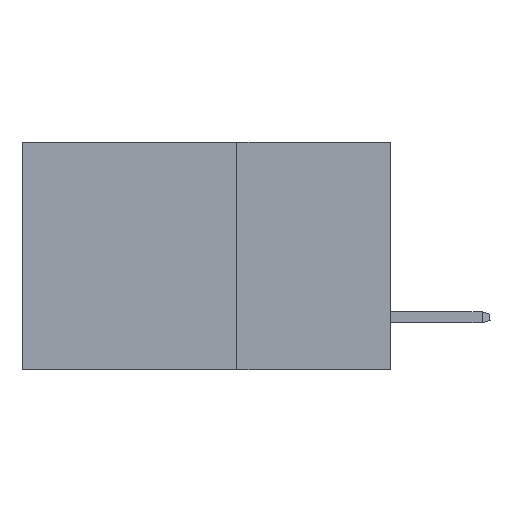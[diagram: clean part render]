
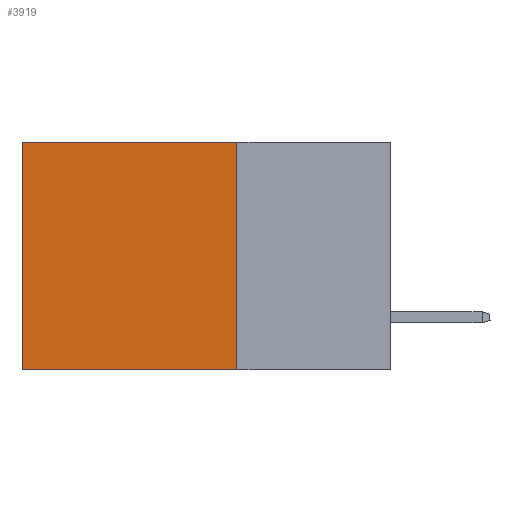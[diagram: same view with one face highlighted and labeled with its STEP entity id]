
A CAD part, left-side view. The second image highlights one B-rep face of the part: STEP entity #3919.
In plain terms, the highlighted planar face has unit normal (-1, 0, 0).
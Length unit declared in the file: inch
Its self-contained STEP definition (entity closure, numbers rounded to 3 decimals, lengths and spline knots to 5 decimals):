
#360 = VECTOR ( 'NONE', #10795, 39.37008 ) ;
#490 = VERTEX_POINT ( 'NONE', #14392 ) ;
#1005 = DIRECTION ( 'NONE',  ( 0., 1., 0. ) ) ;
#1108 = ORIENTED_EDGE ( 'NONE', *, *, #11554, .T. ) ;
#1301 = CARTESIAN_POINT ( 'NONE',  ( 0.2875, 0.6, 0. ) ) ;
#2172 = CARTESIAN_POINT ( 'NONE',  ( 0.2875, 0.25, -0.37 ) ) ;
#2289 = ORIENTED_EDGE ( 'NONE', *, *, #12876, .F. ) ;
#2395 = VECTOR ( 'NONE', #13802, 39.37008 ) ;
#2770 = VERTEX_POINT ( 'NONE', #1301 ) ;
#3777 = CARTESIAN_POINT ( 'NONE',  ( 0.2875, 0.25, 0. ) ) ;
#3919 = ADVANCED_FACE ( 'NONE', ( #8618 ), #6245, .F. ) ;
#4051 = CARTESIAN_POINT ( 'NONE',  ( 0.2875, 0.6, 0. ) ) ;
#4316 = CARTESIAN_POINT ( 'NONE',  ( 0.2875, 0.6, -0.37 ) ) ;
#5321 = ORIENTED_EDGE ( 'NONE', *, *, #7747, .F. ) ;
#5428 = VECTOR ( 'NONE', #7438, 39.37008 ) ;
#5544 = AXIS2_PLACEMENT_3D ( 'NONE', #9709, #6350, #14471 ) ;
#5900 = EDGE_CURVE ( 'NONE', #10253, #2770, #9810, .T. ) ;
#6245 = PLANE ( 'NONE',  #5544 ) ;
#6297 = LINE ( 'NONE', #2172, #9583 ) ;
#6350 = DIRECTION ( 'NONE',  ( 1., 0., 0. ) ) ;
#6803 = CARTESIAN_POINT ( 'NONE',  ( 0.2875, 0.25, 0. ) ) ;
#6838 = CARTESIAN_POINT ( 'NONE',  ( 0.2875, 0.25, 0. ) ) ;
#7438 = DIRECTION ( 'NONE',  ( 0., 0., -1. ) ) ;
#7747 = EDGE_CURVE ( 'NONE', #490, #12431, #6297, .T. ) ;
#8618 = FACE_OUTER_BOUND ( 'NONE', #14784, .T. ) ;
#9583 = VECTOR ( 'NONE', #1005, 39.37008 ) ;
#9709 = CARTESIAN_POINT ( 'NONE',  ( 0.2875, 0.25, 0. ) ) ;
#9810 = LINE ( 'NONE', #6838, #2395 ) ;
#10253 = VERTEX_POINT ( 'NONE', #6803 ) ;
#10795 = DIRECTION ( 'NONE',  ( 0., 0., -1. ) ) ;
#11554 = EDGE_CURVE ( 'NONE', #2770, #12431, #13951, .T. ) ;
#12251 = LINE ( 'NONE', #3777, #360 ) ;
#12431 = VERTEX_POINT ( 'NONE', #4316 ) ;
#12876 = EDGE_CURVE ( 'NONE', #10253, #490, #12251, .T. ) ;
#13802 = DIRECTION ( 'NONE',  ( 0., 1., 0. ) ) ;
#13951 = LINE ( 'NONE', #4051, #5428 ) ;
#14392 = CARTESIAN_POINT ( 'NONE',  ( 0.2875, 0.25, -0.37 ) ) ;
#14454 = ORIENTED_EDGE ( 'NONE', *, *, #5900, .T. ) ;
#14471 = DIRECTION ( 'NONE',  ( 0., 0., -1. ) ) ;
#14784 = EDGE_LOOP ( 'NONE', ( #1108, #5321, #2289, #14454 ) ) ;
